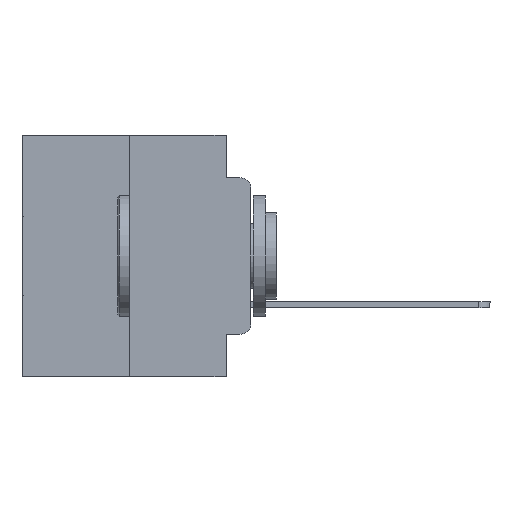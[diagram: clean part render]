
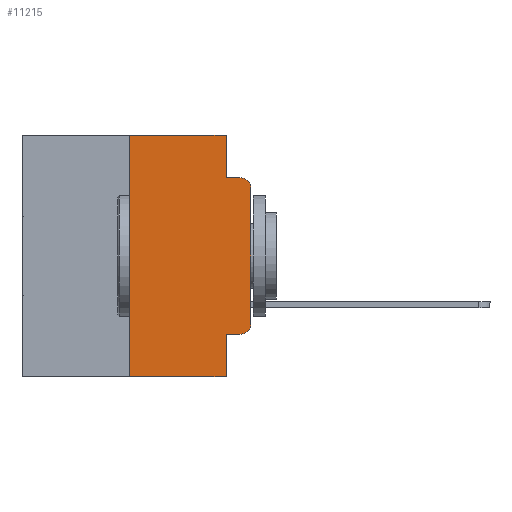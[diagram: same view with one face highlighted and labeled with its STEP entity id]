
A CAD part, left-side view. The second image highlights one B-rep face of the part: STEP entity #11215.
In plain terms, the highlighted planar face has unit normal (-1, 0, 0).
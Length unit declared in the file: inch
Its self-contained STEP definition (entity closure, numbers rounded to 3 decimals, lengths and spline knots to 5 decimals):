
#147 = EDGE_CURVE ( 'NONE', #11406, #10770, #3229, .T. ) ;
#1026 = AXIS2_PLACEMENT_3D ( 'NONE', #24734, #27046, #29022 ) ;
#1477 = CARTESIAN_POINT ( 'NONE',  ( 0., 0.25, 0. ) ) ;
#1861 = DIRECTION ( 'NONE',  ( 0., -1., 0. ) ) ;
#2603 = CARTESIAN_POINT ( 'NONE',  ( 0., 0.25, -0.5 ) ) ;
#2937 = EDGE_CURVE ( 'NONE', #10604, #20202, #19391, .T. ) ;
#3229 = LINE ( 'NONE', #21933, #9447 ) ;
#3587 = VERTEX_POINT ( 'NONE', #9022 ) ;
#3665 = CARTESIAN_POINT ( 'NONE',  ( 0., 0.02, -0.0885 ) ) ;
#3685 = VERTEX_POINT ( 'NONE', #16589 ) ;
#3977 = VERTEX_POINT ( 'NONE', #29583 ) ;
#4230 = EDGE_CURVE ( 'NONE', #10770, #20446, #14208, .T. ) ;
#4637 = CARTESIAN_POINT ( 'NONE',  ( 0., 0.25, 0. ) ) ;
#4738 = CARTESIAN_POINT ( 'NONE',  ( 0., 0.051, -0.0885 ) ) ;
#4807 = LINE ( 'NONE', #14257, #5934 ) ;
#5285 = DIRECTION ( 'NONE',  ( 0., 0., 1. ) ) ;
#5934 = VECTOR ( 'NONE', #23639, 39.37008 ) ;
#6344 = CARTESIAN_POINT ( 'NONE',  ( 0., 0.051, -0.4115 ) ) ;
#6923 = VERTEX_POINT ( 'NONE', #2603 ) ;
#7565 = AXIS2_PLACEMENT_3D ( 'NONE', #26349, #10024, #14657 ) ;
#8233 = ORIENTED_EDGE ( 'NONE', *, *, #4230, .F. ) ;
#8757 = EDGE_LOOP ( 'NONE', ( #22696, #12900, #21835, #8233, #20689, #9012, #12407, #23041, #10217, #16716 ) ) ;
#9012 = ORIENTED_EDGE ( 'NONE', *, *, #10622, .F. ) ;
#9022 = CARTESIAN_POINT ( 'NONE',  ( 0., 0.051, -0.5 ) ) ;
#9371 = VECTOR ( 'NONE', #27707, 39.37008 ) ;
#9397 = CARTESIAN_POINT ( 'NONE',  ( 0., 0.473, 0. ) ) ;
#9447 = VECTOR ( 'NONE', #14838, 39.37008 ) ;
#9541 = DIRECTION ( 'NONE',  ( 0., -1., 0. ) ) ;
#9555 = FACE_OUTER_BOUND ( 'NONE', #8757, .T. ) ;
#10024 = DIRECTION ( 'NONE',  ( -1., 0., 0. ) ) ;
#10099 = LINE ( 'NONE', #26105, #20180 ) ;
#10217 = ORIENTED_EDGE ( 'NONE', *, *, #29466, .T. ) ;
#10604 = VERTEX_POINT ( 'NONE', #20411 ) ;
#10622 = EDGE_CURVE ( 'NONE', #6923, #11406, #25753, .T. ) ;
#10770 = VERTEX_POINT ( 'NONE', #19168 ) ;
#11215 = ADVANCED_FACE ( 'NONE', ( #9555 ), #28479, .F. ) ;
#11406 = VERTEX_POINT ( 'NONE', #1477 ) ;
#12025 = LINE ( 'NONE', #4738, #15851 ) ;
#12407 = ORIENTED_EDGE ( 'NONE', *, *, #17030, .T. ) ;
#12900 = ORIENTED_EDGE ( 'NONE', *, *, #2937, .T. ) ;
#12906 = CARTESIAN_POINT ( 'NONE',  ( 0., 0.051, -0.0885 ) ) ;
#14208 = LINE ( 'NONE', #28798, #17448 ) ;
#14257 = CARTESIAN_POINT ( 'NONE',  ( 0., 0.051, 0. ) ) ;
#14349 = DIRECTION ( 'NONE',  ( 0., 0., -1. ) ) ;
#14657 = DIRECTION ( 'NONE',  ( 0., 0., -1. ) ) ;
#14664 = DIRECTION ( 'NONE',  ( 0., 0., -1. ) ) ;
#14838 = DIRECTION ( 'NONE',  ( 0., -1., 0. ) ) ;
#15360 = CIRCLE ( 'NONE', #1026, 0.02 ) ;
#15851 = VECTOR ( 'NONE', #9541, 39.37008 ) ;
#15930 = LINE ( 'NONE', #6344, #25875 ) ;
#16012 = EDGE_CURVE ( 'NONE', #3977, #10604, #10099, .T. ) ;
#16352 = DIRECTION ( 'NONE',  ( 1., 0., 0. ) ) ;
#16589 = CARTESIAN_POINT ( 'NONE',  ( 0., 0.02, -0.4115 ) ) ;
#16716 = ORIENTED_EDGE ( 'NONE', *, *, #17830, .T. ) ;
#17030 = EDGE_CURVE ( 'NONE', #6923, #3587, #18646, .T. ) ;
#17448 = VECTOR ( 'NONE', #14664, 39.37008 ) ;
#17830 = EDGE_CURVE ( 'NONE', #3685, #3977, #15360, .T. ) ;
#18155 = EDGE_CURVE ( 'NONE', #29968, #3587, #4807, .T. ) ;
#18333 = CARTESIAN_POINT ( 'NONE',  ( 0., 0.473, -0.5 ) ) ;
#18646 = LINE ( 'NONE', #18333, #9371 ) ;
#19168 = CARTESIAN_POINT ( 'NONE',  ( 0., 0.051, 0. ) ) ;
#19391 = CIRCLE ( 'NONE', #7565, 0.02 ) ;
#20180 = VECTOR ( 'NONE', #5285, 39.37008 ) ;
#20202 = VERTEX_POINT ( 'NONE', #3665 ) ;
#20411 = CARTESIAN_POINT ( 'NONE',  ( 0., 0., -0.1085 ) ) ;
#20446 = VERTEX_POINT ( 'NONE', #12906 ) ;
#20489 = AXIS2_PLACEMENT_3D ( 'NONE', #9397, #16352, #14349 ) ;
#20689 = ORIENTED_EDGE ( 'NONE', *, *, #147, .F. ) ;
#21835 = ORIENTED_EDGE ( 'NONE', *, *, #23666, .F. ) ;
#21933 = CARTESIAN_POINT ( 'NONE',  ( 0., 0.473, 0. ) ) ;
#22696 = ORIENTED_EDGE ( 'NONE', *, *, #16012, .T. ) ;
#23041 = ORIENTED_EDGE ( 'NONE', *, *, #18155, .F. ) ;
#23639 = DIRECTION ( 'NONE',  ( 0., 0., -1. ) ) ;
#23666 = EDGE_CURVE ( 'NONE', #20446, #20202, #12025, .T. ) ;
#23911 = VECTOR ( 'NONE', #29903, 39.37008 ) ;
#24734 = CARTESIAN_POINT ( 'NONE',  ( 0., 0.02, -0.3915 ) ) ;
#25424 = CARTESIAN_POINT ( 'NONE',  ( 0., 0.051, -0.4115 ) ) ;
#25753 = LINE ( 'NONE', #4637, #23911 ) ;
#25875 = VECTOR ( 'NONE', #1861, 39.37008 ) ;
#26105 = CARTESIAN_POINT ( 'NONE',  ( 0., 0., 0. ) ) ;
#26349 = CARTESIAN_POINT ( 'NONE',  ( 0., 0.02, -0.1085 ) ) ;
#27046 = DIRECTION ( 'NONE',  ( -1., 0., 0. ) ) ;
#27707 = DIRECTION ( 'NONE',  ( 0., -1., 0. ) ) ;
#28479 = PLANE ( 'NONE',  #20489 ) ;
#28798 = CARTESIAN_POINT ( 'NONE',  ( 0., 0.051, 0. ) ) ;
#29022 = DIRECTION ( 'NONE',  ( 0., 0., -1. ) ) ;
#29466 = EDGE_CURVE ( 'NONE', #29968, #3685, #15930, .T. ) ;
#29583 = CARTESIAN_POINT ( 'NONE',  ( 0., 0., -0.3915 ) ) ;
#29903 = DIRECTION ( 'NONE',  ( 0., 0., 1. ) ) ;
#29968 = VERTEX_POINT ( 'NONE', #25424 ) ;
